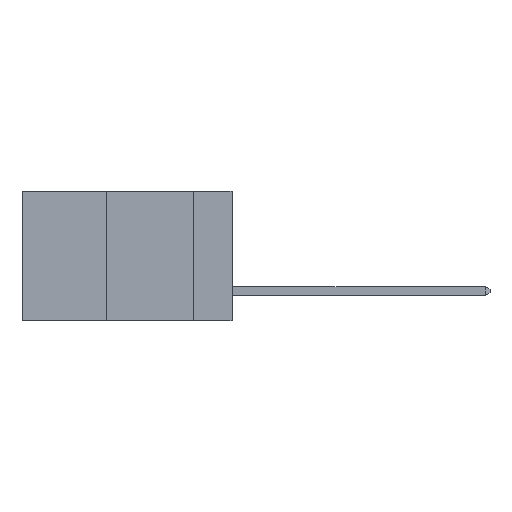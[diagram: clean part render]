
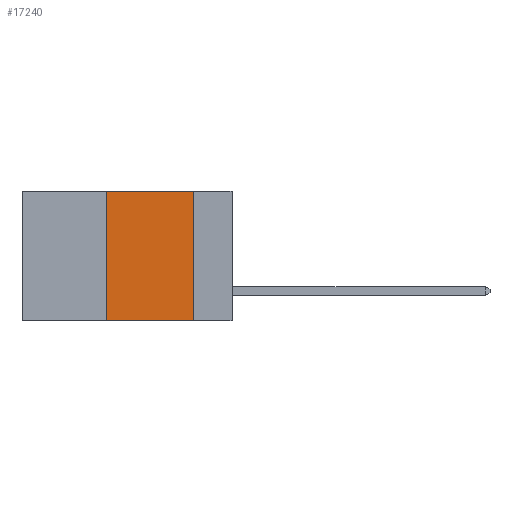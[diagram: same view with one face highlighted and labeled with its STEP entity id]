
A CAD part, left-side view. The second image highlights one B-rep face of the part: STEP entity #17240.
In plain terms, the highlighted planar face has unit normal (-1, 0, 0).
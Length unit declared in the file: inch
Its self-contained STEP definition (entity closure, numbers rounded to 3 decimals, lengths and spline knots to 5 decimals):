
#101 = EDGE_CURVE ( 'NONE', #16634, #21724, #16910, .T. ) ;
#279 = CARTESIAN_POINT ( 'NONE',  ( 0., 0.6, -0.37 ) ) ;
#784 = ORIENTED_EDGE ( 'NONE', *, *, #26706, .T. ) ;
#3726 = FACE_OUTER_BOUND ( 'NONE', #16092, .T. ) ;
#4975 = DIRECTION ( 'NONE',  ( 0., 0., 1. ) ) ;
#5582 = VERTEX_POINT ( 'NONE', #28809 ) ;
#7639 = CARTESIAN_POINT ( 'NONE',  ( 0., 0.36, 0. ) ) ;
#12064 = CARTESIAN_POINT ( 'NONE',  ( 0., 0.6, 0. ) ) ;
#12089 = DIRECTION ( 'NONE',  ( 0., -1., 0. ) ) ;
#13529 = CARTESIAN_POINT ( 'NONE',  ( 0., 0.6, 0. ) ) ;
#14860 = DIRECTION ( 'NONE',  ( 0., 0., -1. ) ) ;
#16029 = VECTOR ( 'NONE', #12089, 39.37008 ) ;
#16092 = EDGE_LOOP ( 'NONE', ( #35840, #28673, #31927, #784 ) ) ;
#16297 = VECTOR ( 'NONE', #17138, 39.37008 ) ;
#16634 = VERTEX_POINT ( 'NONE', #31430 ) ;
#16910 = LINE ( 'NONE', #13529, #16029 ) ;
#17138 = DIRECTION ( 'NONE',  ( 0., -1., 0. ) ) ;
#17168 = LINE ( 'NONE', #279, #16297 ) ;
#17240 = ADVANCED_FACE ( 'NONE', ( #3726 ), #25791, .F. ) ;
#17376 = CARTESIAN_POINT ( 'NONE',  ( 0., 0.36, -0.37 ) ) ;
#21724 = VERTEX_POINT ( 'NONE', #34031 ) ;
#24688 = VECTOR ( 'NONE', #4975, 39.37008 ) ;
#24717 = DIRECTION ( 'NONE',  ( 0., 0., -1. ) ) ;
#25101 = VECTOR ( 'NONE', #24717, 39.37008 ) ;
#25791 = PLANE ( 'NONE',  #33817 ) ;
#26706 = EDGE_CURVE ( 'NONE', #30772, #5582, #17168, .T. ) ;
#28528 = EDGE_CURVE ( 'NONE', #21724, #5582, #32356, .T. ) ;
#28673 = ORIENTED_EDGE ( 'NONE', *, *, #101, .F. ) ;
#28809 = CARTESIAN_POINT ( 'NONE',  ( 0., 0.11, -0.37 ) ) ;
#30772 = VERTEX_POINT ( 'NONE', #17376 ) ;
#31267 = DIRECTION ( 'NONE',  ( 1., 0., 0. ) ) ;
#31430 = CARTESIAN_POINT ( 'NONE',  ( 0., 0.36, 0. ) ) ;
#31927 = ORIENTED_EDGE ( 'NONE', *, *, #35816, .F. ) ;
#32356 = LINE ( 'NONE', #35527, #25101 ) ;
#32793 = LINE ( 'NONE', #7639, #24688 ) ;
#33817 = AXIS2_PLACEMENT_3D ( 'NONE', #12064, #31267, #14860 ) ;
#34031 = CARTESIAN_POINT ( 'NONE',  ( 0., 0.11, 0. ) ) ;
#35527 = CARTESIAN_POINT ( 'NONE',  ( 0., 0.11, 0. ) ) ;
#35816 = EDGE_CURVE ( 'NONE', #30772, #16634, #32793, .T. ) ;
#35840 = ORIENTED_EDGE ( 'NONE', *, *, #28528, .F. ) ;
